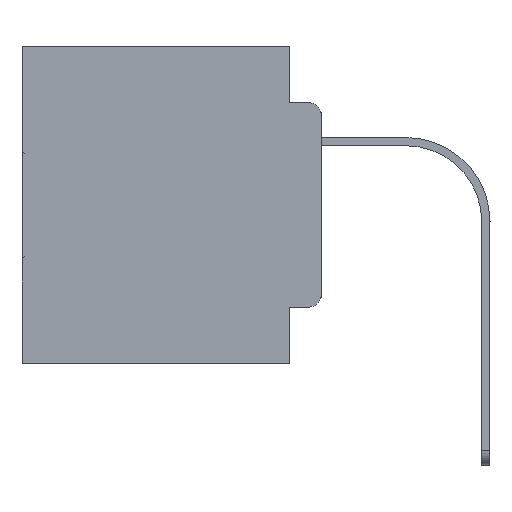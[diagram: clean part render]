
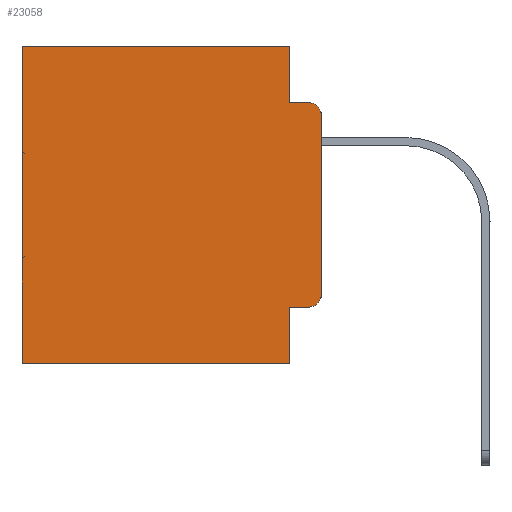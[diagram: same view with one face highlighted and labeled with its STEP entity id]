
A CAD part, left-side view. The second image highlights one B-rep face of the part: STEP entity #23058.
In plain terms, the highlighted planar face has unit normal (-1, 0, 0).
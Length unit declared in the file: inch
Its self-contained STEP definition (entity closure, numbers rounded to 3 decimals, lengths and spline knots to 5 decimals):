
#175 = CARTESIAN_POINT ( 'NONE',  ( 0.298, 0., -0.1085 ) ) ;
#284 = CIRCLE ( 'NONE', #27216, 0.02 ) ;
#414 = CARTESIAN_POINT ( 'NONE',  ( 0.298, 0., 0. ) ) ;
#853 = ORIENTED_EDGE ( 'NONE', *, *, #15003, .T. ) ;
#1104 = CARTESIAN_POINT ( 'NONE',  ( 0.298, 0., -0.3915 ) ) ;
#1204 = VERTEX_POINT ( 'NONE', #1104 ) ;
#1487 = ORIENTED_EDGE ( 'NONE', *, *, #14531, .F. ) ;
#1829 = CARTESIAN_POINT ( 'NONE',  ( 0.298, 0.473, 0. ) ) ;
#1833 = CARTESIAN_POINT ( 'NONE',  ( 0.298, 0.051, -0.4115 ) ) ;
#2076 = EDGE_CURVE ( 'NONE', #3050, #7644, #24265, .T. ) ;
#2470 = DIRECTION ( 'NONE',  ( 0., 1., 0. ) ) ;
#2832 = EDGE_CURVE ( 'NONE', #6206, #1204, #284, .T. ) ;
#3046 = VECTOR ( 'NONE', #28949, 39.37008 ) ;
#3050 = VERTEX_POINT ( 'NONE', #23163 ) ;
#3747 = DIRECTION ( 'NONE',  ( 0., -1., 0. ) ) ;
#3907 = CARTESIAN_POINT ( 'NONE',  ( 0.298, 0.473, 0. ) ) ;
#4426 = CARTESIAN_POINT ( 'NONE',  ( 0.298, 0.051, -0.4115 ) ) ;
#4731 = VERTEX_POINT ( 'NONE', #29980 ) ;
#5538 = EDGE_CURVE ( 'NONE', #13500, #13918, #24633, .T. ) ;
#5693 = CARTESIAN_POINT ( 'NONE',  ( 0.298, 0.051, -0.5 ) ) ;
#5759 = ORIENTED_EDGE ( 'NONE', *, *, #7668, .T. ) ;
#6163 = EDGE_CURVE ( 'NONE', #3050, #12683, #12817, .T. ) ;
#6206 = VERTEX_POINT ( 'NONE', #18058 ) ;
#6251 = DIRECTION ( 'NONE',  ( -1., 0., 0. ) ) ;
#6539 = ORIENTED_EDGE ( 'NONE', *, *, #2076, .T. ) ;
#6833 = VECTOR ( 'NONE', #8824, 39.37008 ) ;
#6926 = DIRECTION ( 'NONE',  ( 1., 0., 0. ) ) ;
#6969 = CARTESIAN_POINT ( 'NONE',  ( 0.298, 0.02, -0.1085 ) ) ;
#7350 = ORIENTED_EDGE ( 'NONE', *, *, #6163, .F. ) ;
#7474 = AXIS2_PLACEMENT_3D ( 'NONE', #6969, #28606, #23367 ) ;
#7644 = VERTEX_POINT ( 'NONE', #1829 ) ;
#7668 = EDGE_CURVE ( 'NONE', #7644, #13918, #30620, .T. ) ;
#7942 = ORIENTED_EDGE ( 'NONE', *, *, #17656, .F. ) ;
#8456 = ORIENTED_EDGE ( 'NONE', *, *, #27657, .F. ) ;
#8824 = DIRECTION ( 'NONE',  ( 0., 0., -1. ) ) ;
#9092 = CARTESIAN_POINT ( 'NONE',  ( 0.298, 0.051, 0. ) ) ;
#9491 = CARTESIAN_POINT ( 'NONE',  ( 0.298, 0., 0. ) ) ;
#10109 = DIRECTION ( 'NONE',  ( 0., 0., -1. ) ) ;
#11074 = LINE ( 'NONE', #15992, #28759 ) ;
#11878 = EDGE_CURVE ( 'NONE', #13636, #6206, #20778, .T. ) ;
#11931 = CARTESIAN_POINT ( 'NONE',  ( 0.298, 0., -0.5 ) ) ;
#11955 = DIRECTION ( 'NONE',  ( 0., 0., -1. ) ) ;
#12089 = CIRCLE ( 'NONE', #7474, 0.02 ) ;
#12186 = CARTESIAN_POINT ( 'NONE',  ( 0.298, 0., 0. ) ) ;
#12683 = VERTEX_POINT ( 'NONE', #17948 ) ;
#12817 = LINE ( 'NONE', #29836, #21828 ) ;
#13291 = DIRECTION ( 'NONE',  ( 0., -1., 0. ) ) ;
#13500 = VERTEX_POINT ( 'NONE', #5693 ) ;
#13636 = VERTEX_POINT ( 'NONE', #4426 ) ;
#13918 = VERTEX_POINT ( 'NONE', #18077 ) ;
#14531 = EDGE_CURVE ( 'NONE', #13636, #13500, #30716, .T. ) ;
#15003 = EDGE_CURVE ( 'NONE', #23969, #4731, #12089, .T. ) ;
#15992 = CARTESIAN_POINT ( 'NONE',  ( 0.298, 0.051, -0.0885 ) ) ;
#17425 = VECTOR ( 'NONE', #2470, 39.37008 ) ;
#17656 = EDGE_CURVE ( 'NONE', #23969, #1204, #29357, .T. ) ;
#17928 = ORIENTED_EDGE ( 'NONE', *, *, #11878, .T. ) ;
#17948 = CARTESIAN_POINT ( 'NONE',  ( 0.298, 0.051, -0.0885 ) ) ;
#18058 = CARTESIAN_POINT ( 'NONE',  ( 0.298, 0.02, -0.4115 ) ) ;
#18077 = CARTESIAN_POINT ( 'NONE',  ( 0.298, 0.473, -0.5 ) ) ;
#18455 = ORIENTED_EDGE ( 'NONE', *, *, #5538, .F. ) ;
#18656 = CARTESIAN_POINT ( 'NONE',  ( 0.298, 0.02, -0.3915 ) ) ;
#19015 = FACE_OUTER_BOUND ( 'NONE', #23309, .T. ) ;
#20778 = LINE ( 'NONE', #1833, #22592 ) ;
#21828 = VECTOR ( 'NONE', #27147, 39.37008 ) ;
#21885 = PLANE ( 'NONE',  #23915 ) ;
#22592 = VECTOR ( 'NONE', #3747, 39.37008 ) ;
#23058 = ADVANCED_FACE ( 'NONE', ( #19015 ), #21885, .F. ) ;
#23163 = CARTESIAN_POINT ( 'NONE',  ( 0.298, 0.051, 0. ) ) ;
#23309 = EDGE_LOOP ( 'NONE', ( #7942, #853, #8456, #7350, #6539, #5759, #18455, #1487, #17928, #25141 ) ) ;
#23367 = DIRECTION ( 'NONE',  ( 0., 0., -1. ) ) ;
#23427 = DIRECTION ( 'NONE',  ( 0., 0., -1. ) ) ;
#23915 = AXIS2_PLACEMENT_3D ( 'NONE', #9491, #6926, #29192 ) ;
#23969 = VERTEX_POINT ( 'NONE', #175 ) ;
#24265 = LINE ( 'NONE', #12186, #17425 ) ;
#24633 = LINE ( 'NONE', #11931, #3046 ) ;
#25141 = ORIENTED_EDGE ( 'NONE', *, *, #2832, .T. ) ;
#27147 = DIRECTION ( 'NONE',  ( 0., 0., -1. ) ) ;
#27216 = AXIS2_PLACEMENT_3D ( 'NONE', #18656, #6251, #23427 ) ;
#27657 = EDGE_CURVE ( 'NONE', #12683, #4731, #11074, .T. ) ;
#27843 = VECTOR ( 'NONE', #11955, 39.37008 ) ;
#28242 = VECTOR ( 'NONE', #10109, 39.37008 ) ;
#28606 = DIRECTION ( 'NONE',  ( -1., 0., 0. ) ) ;
#28759 = VECTOR ( 'NONE', #13291, 39.37008 ) ;
#28949 = DIRECTION ( 'NONE',  ( 0., 1., 0. ) ) ;
#29192 = DIRECTION ( 'NONE',  ( 0., 0., -1. ) ) ;
#29357 = LINE ( 'NONE', #414, #28242 ) ;
#29836 = CARTESIAN_POINT ( 'NONE',  ( 0.298, 0.051, 0. ) ) ;
#29980 = CARTESIAN_POINT ( 'NONE',  ( 0.298, 0.02, -0.0885 ) ) ;
#30620 = LINE ( 'NONE', #3907, #6833 ) ;
#30716 = LINE ( 'NONE', #9092, #27843 ) ;
